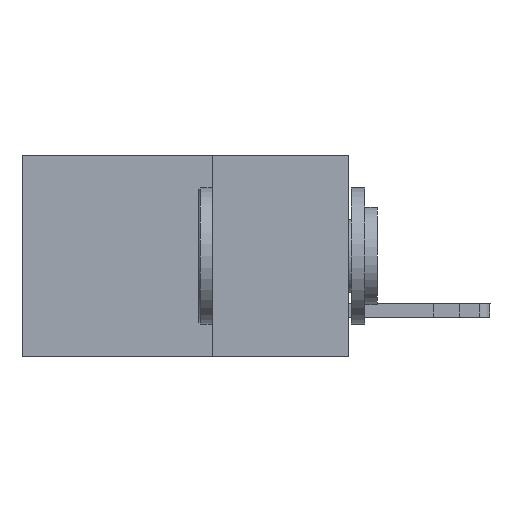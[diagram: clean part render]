
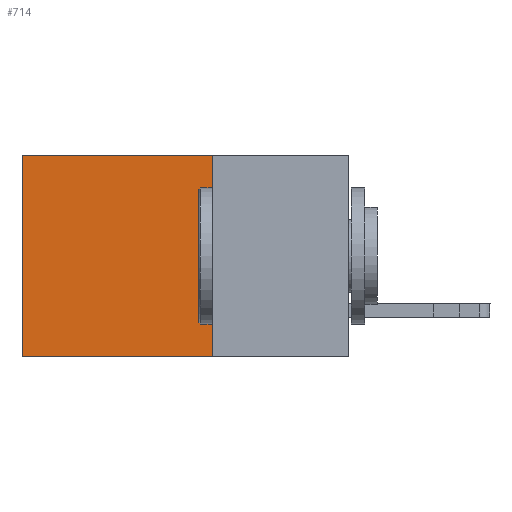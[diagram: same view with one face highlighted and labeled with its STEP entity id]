
A CAD part, left-side view. The second image highlights one B-rep face of the part: STEP entity #714.
In plain terms, the highlighted planar face has unit normal (-1, 0, 0).
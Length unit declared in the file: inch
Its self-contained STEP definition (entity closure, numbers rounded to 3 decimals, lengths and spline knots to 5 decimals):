
#30 = VERTEX_POINT ( 'NONE', #3457 ) ;
#82 = EDGE_CURVE ( 'NONE', #7975, #6654, #2598, .T. ) ;
#714 = ADVANCED_FACE ( 'NONE', ( #8576 ), #3665, .F. ) ;
#986 = ORIENTED_EDGE ( 'NONE', *, *, #8545, .T. ) ;
#1692 = VECTOR ( 'NONE', #8318, 39.37008 ) ;
#2598 = LINE ( 'NONE', #11498, #8754 ) ;
#2780 = DIRECTION ( 'NONE',  ( 1., 0., 0. ) ) ;
#3387 = VERTEX_POINT ( 'NONE', #4195 ) ;
#3457 = CARTESIAN_POINT ( 'NONE',  ( 0.298, 0.6, -0.37 ) ) ;
#3665 = PLANE ( 'NONE',  #5498 ) ;
#4195 = CARTESIAN_POINT ( 'NONE',  ( 0.298, 0.6, 0. ) ) ;
#4534 = CARTESIAN_POINT ( 'NONE',  ( 0.298, 0.25, 0. ) ) ;
#4708 = CARTESIAN_POINT ( 'NONE',  ( 0.298, 0.25, -0.37 ) ) ;
#4744 = DIRECTION ( 'NONE',  ( 0., 1., 0. ) ) ;
#4749 = ORIENTED_EDGE ( 'NONE', *, *, #82, .F. ) ;
#5337 = VECTOR ( 'NONE', #4744, 39.37008 ) ;
#5498 = AXIS2_PLACEMENT_3D ( 'NONE', #12592, #2780, #7770 ) ;
#5619 = VECTOR ( 'NONE', #7448, 39.37008 ) ;
#5941 = ORIENTED_EDGE ( 'NONE', *, *, #10812, .F. ) ;
#6654 = VERTEX_POINT ( 'NONE', #6794 ) ;
#6794 = CARTESIAN_POINT ( 'NONE',  ( 0.298, 0.25, -0.37 ) ) ;
#7154 = LINE ( 'NONE', #4708, #5337 ) ;
#7448 = DIRECTION ( 'NONE',  ( 0., 0., -1. ) ) ;
#7492 = CARTESIAN_POINT ( 'NONE',  ( 0.298, 0.6, 0. ) ) ;
#7770 = DIRECTION ( 'NONE',  ( 0., 0., -1. ) ) ;
#7975 = VERTEX_POINT ( 'NONE', #12331 ) ;
#8192 = LINE ( 'NONE', #7492, #5619 ) ;
#8318 = DIRECTION ( 'NONE',  ( 0., 1., 0. ) ) ;
#8545 = EDGE_CURVE ( 'NONE', #7975, #3387, #10917, .T. ) ;
#8576 = FACE_OUTER_BOUND ( 'NONE', #10065, .T. ) ;
#8754 = VECTOR ( 'NONE', #9598, 39.37008 ) ;
#9598 = DIRECTION ( 'NONE',  ( 0., 0., -1. ) ) ;
#10065 = EDGE_LOOP ( 'NONE', ( #11473, #5941, #4749, #986 ) ) ;
#10812 = EDGE_CURVE ( 'NONE', #6654, #30, #7154, .T. ) ;
#10917 = LINE ( 'NONE', #4534, #1692 ) ;
#11285 = EDGE_CURVE ( 'NONE', #3387, #30, #8192, .T. ) ;
#11473 = ORIENTED_EDGE ( 'NONE', *, *, #11285, .T. ) ;
#11498 = CARTESIAN_POINT ( 'NONE',  ( 0.298, 0.25, 0. ) ) ;
#12331 = CARTESIAN_POINT ( 'NONE',  ( 0.298, 0.25, 0. ) ) ;
#12592 = CARTESIAN_POINT ( 'NONE',  ( 0.298, 0.25, 0. ) ) ;
